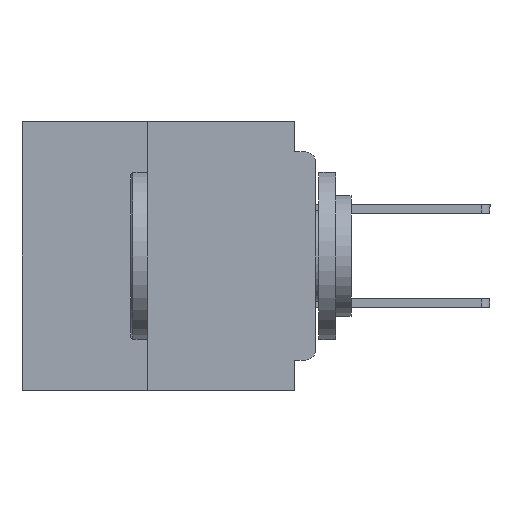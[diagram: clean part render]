
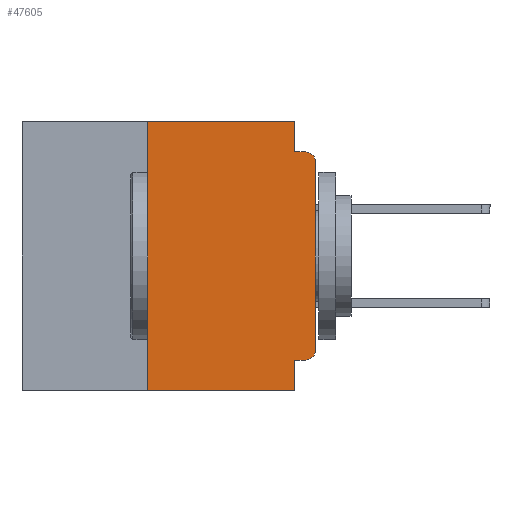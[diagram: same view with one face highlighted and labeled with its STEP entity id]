
A CAD part, left-side view. The second image highlights one B-rep face of the part: STEP entity #47605.
In plain terms, the highlighted planar face has unit normal (-1, 0, 0).
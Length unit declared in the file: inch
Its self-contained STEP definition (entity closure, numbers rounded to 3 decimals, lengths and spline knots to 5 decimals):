
#663 = VERTEX_POINT ( 'NONE', #47524 ) ;
#2024 = VECTOR ( 'NONE', #40585, 39.37008 ) ;
#2216 = CARTESIAN_POINT ( 'NONE',  ( 0., 0., -0.06 ) ) ;
#3088 = EDGE_CURVE ( 'NONE', #12342, #663, #39003, .T. ) ;
#3301 = VERTEX_POINT ( 'NONE', #28127 ) ;
#3557 = ORIENTED_EDGE ( 'NONE', *, *, #3802, .T. ) ;
#3802 = EDGE_CURVE ( 'NONE', #3301, #4580, #27442, .T. ) ;
#4500 = ORIENTED_EDGE ( 'NONE', *, *, #8606, .F. ) ;
#4580 = VERTEX_POINT ( 'NONE', #2216 ) ;
#4735 = CARTESIAN_POINT ( 'NONE',  ( 0., 0.25, -0.4 ) ) ;
#5057 = CARTESIAN_POINT ( 'NONE',  ( 0., 0., -0.045 ) ) ;
#5870 = EDGE_CURVE ( 'NONE', #12342, #26136, #29190, .T. ) ;
#6732 = EDGE_CURVE ( 'NONE', #26136, #40516, #50805, .T. ) ;
#7204 = CARTESIAN_POINT ( 'NONE',  ( 0., 0.031, -0.4 ) ) ;
#7402 = CARTESIAN_POINT ( 'NONE',  ( 0., 0.031, -0.355 ) ) ;
#7875 = VECTOR ( 'NONE', #29379, 39.37008 ) ;
#7885 = DIRECTION ( 'NONE',  ( 0., 1., 0. ) ) ;
#8606 = EDGE_CURVE ( 'NONE', #40516, #9887, #51314, .T. ) ;
#8644 = CIRCLE ( 'NONE', #32850, 0.015 ) ;
#9810 = CARTESIAN_POINT ( 'NONE',  ( 0., 0.031, -0.045 ) ) ;
#9887 = VERTEX_POINT ( 'NONE', #9810 ) ;
#12216 = ORIENTED_EDGE ( 'NONE', *, *, #50458, .F. ) ;
#12325 = ORIENTED_EDGE ( 'NONE', *, *, #14904, .T. ) ;
#12342 = VERTEX_POINT ( 'NONE', #4735 ) ;
#12858 = EDGE_CURVE ( 'NONE', #9887, #45776, #38063, .T. ) ;
#12962 = LINE ( 'NONE', #7204, #2024 ) ;
#13607 = CARTESIAN_POINT ( 'NONE',  ( 0., 0., 0. ) ) ;
#13968 = DIRECTION ( 'NONE',  ( 0., 0., 1. ) ) ;
#14627 = ORIENTED_EDGE ( 'NONE', *, *, #48717, .T. ) ;
#14837 = ORIENTED_EDGE ( 'NONE', *, *, #6732, .F. ) ;
#14904 = EDGE_CURVE ( 'NONE', #21312, #3301, #8644, .T. ) ;
#15305 = DIRECTION ( 'NONE',  ( 0., -1., 0. ) ) ;
#15575 = AXIS2_PLACEMENT_3D ( 'NONE', #18593, #22663, #51216 ) ;
#16070 = CARTESIAN_POINT ( 'NONE',  ( 0., 0.25, 0. ) ) ;
#16625 = CARTESIAN_POINT ( 'NONE',  ( 0., 0.031, 0. ) ) ;
#17191 = CARTESIAN_POINT ( 'NONE',  ( 0., 0.015, -0.06 ) ) ;
#17984 = CARTESIAN_POINT ( 'NONE',  ( 0., 0.015, -0.34 ) ) ;
#18367 = VECTOR ( 'NONE', #46601, 39.37008 ) ;
#18593 = CARTESIAN_POINT ( 'NONE',  ( 0., 0.437, 0. ) ) ;
#18600 = VECTOR ( 'NONE', #32600, 39.37008 ) ;
#21295 = DIRECTION ( 'NONE',  ( 0., 0., -1. ) ) ;
#21312 = VERTEX_POINT ( 'NONE', #40350 ) ;
#22051 = DIRECTION ( 'NONE',  ( 0., 0., -1. ) ) ;
#22659 = CARTESIAN_POINT ( 'NONE',  ( 0., 0.015, -0.045 ) ) ;
#22663 = DIRECTION ( 'NONE',  ( 1., 0., 0. ) ) ;
#23162 = FACE_OUTER_BOUND ( 'NONE', #26997, .T. ) ;
#23851 = ORIENTED_EDGE ( 'NONE', *, *, #5870, .F. ) ;
#25441 = DIRECTION ( 'NONE',  ( 0., -1., 0. ) ) ;
#26136 = VERTEX_POINT ( 'NONE', #16070 ) ;
#26997 = EDGE_LOOP ( 'NONE', ( #3557, #14627, #50740, #4500, #14837, #23851, #52833, #29733, #12216, #12325 ) ) ;
#27442 = LINE ( 'NONE', #13607, #37015 ) ;
#28127 = CARTESIAN_POINT ( 'NONE',  ( 0., 0., -0.34 ) ) ;
#28254 = CARTESIAN_POINT ( 'NONE',  ( 0., 0., -0.355 ) ) ;
#29190 = LINE ( 'NONE', #50535, #18367 ) ;
#29379 = DIRECTION ( 'NONE',  ( 0., 0., -1. ) ) ;
#29733 = ORIENTED_EDGE ( 'NONE', *, *, #39737, .F. ) ;
#31557 = CARTESIAN_POINT ( 'NONE',  ( 0., 0.437, 0. ) ) ;
#32600 = DIRECTION ( 'NONE',  ( 0., -1., 0. ) ) ;
#32618 = CARTESIAN_POINT ( 'NONE',  ( 0., 0.437, -0.4 ) ) ;
#32850 = AXIS2_PLACEMENT_3D ( 'NONE', #17984, #46509, #22051 ) ;
#35161 = VERTEX_POINT ( 'NONE', #7402 ) ;
#36375 = VECTOR ( 'NONE', #7885, 39.37008 ) ;
#36794 = VECTOR ( 'NONE', #25441, 39.37008 ) ;
#37015 = VECTOR ( 'NONE', #13968, 39.37008 ) ;
#37628 = LINE ( 'NONE', #28254, #36375 ) ;
#37759 = CARTESIAN_POINT ( 'NONE',  ( 0., 0.031, 0. ) ) ;
#38063 = LINE ( 'NONE', #5057, #36794 ) ;
#38381 = CIRCLE ( 'NONE', #45308, 0.015 ) ;
#39003 = LINE ( 'NONE', #32618, #18600 ) ;
#39737 = EDGE_CURVE ( 'NONE', #35161, #663, #12962, .T. ) ;
#39941 = VECTOR ( 'NONE', #15305, 39.37008 ) ;
#40350 = CARTESIAN_POINT ( 'NONE',  ( 0., 0.015, -0.355 ) ) ;
#40516 = VERTEX_POINT ( 'NONE', #16625 ) ;
#40585 = DIRECTION ( 'NONE',  ( 0., 0., -1. ) ) ;
#43008 = PLANE ( 'NONE',  #15575 ) ;
#45308 = AXIS2_PLACEMENT_3D ( 'NONE', #17191, #45725, #21295 ) ;
#45725 = DIRECTION ( 'NONE',  ( -1., 0., 0. ) ) ;
#45776 = VERTEX_POINT ( 'NONE', #22659 ) ;
#46509 = DIRECTION ( 'NONE',  ( -1., 0., 0. ) ) ;
#46601 = DIRECTION ( 'NONE',  ( 0., 0., 1. ) ) ;
#47524 = CARTESIAN_POINT ( 'NONE',  ( 0., 0.031, -0.4 ) ) ;
#47605 = ADVANCED_FACE ( 'NONE', ( #23162 ), #43008, .F. ) ;
#48717 = EDGE_CURVE ( 'NONE', #4580, #45776, #38381, .T. ) ;
#50458 = EDGE_CURVE ( 'NONE', #21312, #35161, #37628, .T. ) ;
#50535 = CARTESIAN_POINT ( 'NONE',  ( 0., 0.25, -0.4 ) ) ;
#50740 = ORIENTED_EDGE ( 'NONE', *, *, #12858, .F. ) ;
#50805 = LINE ( 'NONE', #31557, #39941 ) ;
#51216 = DIRECTION ( 'NONE',  ( 0., 0., -1. ) ) ;
#51314 = LINE ( 'NONE', #37759, #7875 ) ;
#52833 = ORIENTED_EDGE ( 'NONE', *, *, #3088, .T. ) ;
